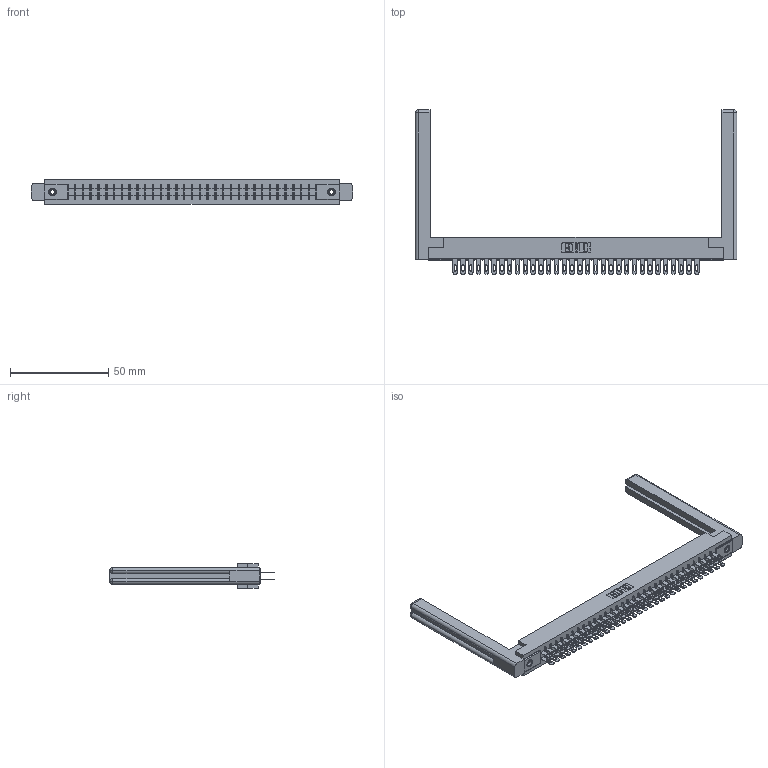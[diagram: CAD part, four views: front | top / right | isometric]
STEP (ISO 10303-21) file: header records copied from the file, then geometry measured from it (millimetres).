
FILE_DESCRIPTION (( 'STEP AP203' ), '1' );
FILE_NAME ('315-064-500-258.STEP', '2019-09-10T20:27:56', ( '' ), ( '' ), 'SwSTEP 2.0', 'SolidWorks 2016', '' );
FILE_SCHEMA (( 'CONFIG_CONTROL_DESIGN' ));
Length unit declared in the file: inch
Products named in the file (5): 345-250-001_345-250-001-102; 315-064-500-258; 305-290-001_500; 305 Part_.156 Dia; 307-220-058
Assembly tree (69 placements, depth 2):
  315-064-500-258
    305 Part_.156 Dia
    305-290-001_500  x64
    345-250-001_345-250-001-102  x2
    307-220-058  x2
Bounding box: 163.42 x 83.49 x 12.7 mm (x, y, z)
Volume: 24346.8 mm3; surface area: 27743.5 mm2
Topology: 69 solids, 69 shells, 3458 faces, 9854 edges, 6384 vertices
Faces by surface type: plane 1944, cylinder 1362, sphere 128, cone 12, torus 12
Entity records: 38520 total; most frequent: CARTESIAN_POINT 6389, ORIENTED_EDGE 6282, DIRECTION 6153, EDGE_CURVE 3141, VECTOR 2517, LINE 2517, VERTEX_POINT 2000, AXIS2_PLACEMENT_3D 1818
